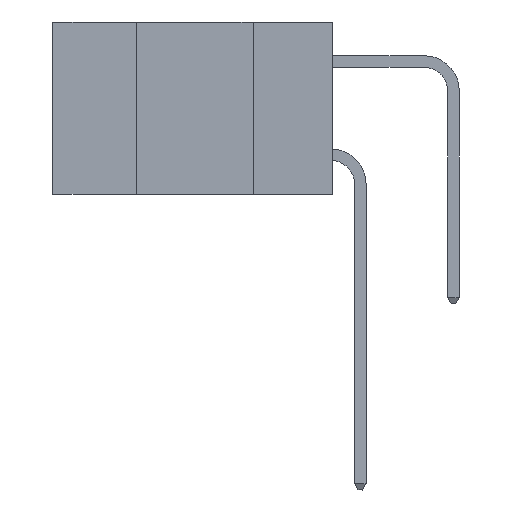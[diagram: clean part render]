
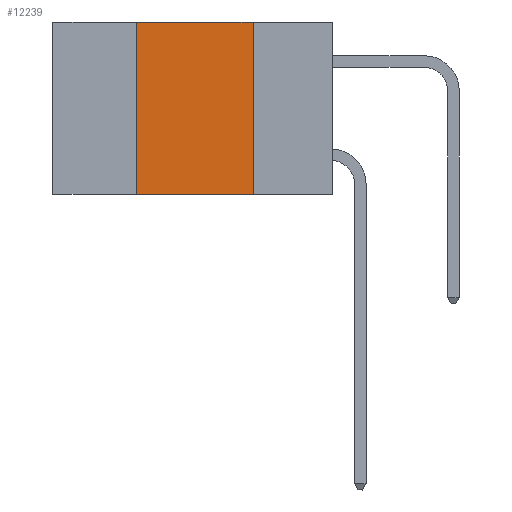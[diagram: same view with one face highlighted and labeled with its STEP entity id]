
A CAD part, left-side view. The second image highlights one B-rep face of the part: STEP entity #12239.
In plain terms, the highlighted planar face has unit normal (-1, 0, 0).
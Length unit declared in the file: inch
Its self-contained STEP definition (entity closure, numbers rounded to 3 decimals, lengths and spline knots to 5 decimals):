
#1234 = LINE ( 'NONE', #1240, #11062 ) ;
#1240 = CARTESIAN_POINT ( 'NONE',  ( 0., 0.6, 0. ) ) ;
#1468 = PLANE ( 'NONE',  #9001 ) ;
#1554 = DIRECTION ( 'NONE',  ( 1., 0., 0. ) ) ;
#2199 = CARTESIAN_POINT ( 'NONE',  ( 0., 0.17, 0. ) ) ;
#2870 = LINE ( 'NONE', #2199, #9507 ) ;
#2906 = CARTESIAN_POINT ( 'NONE',  ( 0., 0.17, 0. ) ) ;
#3190 = DIRECTION ( 'NONE',  ( 0., -1., 0. ) ) ;
#3213 = FACE_OUTER_BOUND ( 'NONE', #6669, .T. ) ;
#3235 = VERTEX_POINT ( 'NONE', #6755 ) ;
#3280 = EDGE_CURVE ( 'NONE', #3368, #3235, #6231, .T. ) ;
#3368 = VERTEX_POINT ( 'NONE', #7272 ) ;
#3686 = VECTOR ( 'NONE', #4241, 39.37008 ) ;
#4083 = LINE ( 'NONE', #10897, #7244 ) ;
#4128 = DIRECTION ( 'NONE',  ( 0., -1., 0. ) ) ;
#4241 = DIRECTION ( 'NONE',  ( 0., 0., 1. ) ) ;
#4661 = CARTESIAN_POINT ( 'NONE',  ( 0., 0.17, -0.37 ) ) ;
#4807 = ORIENTED_EDGE ( 'NONE', *, *, #7144, .F. ) ;
#6231 = LINE ( 'NONE', #9944, #3686 ) ;
#6379 = ORIENTED_EDGE ( 'NONE', *, *, #8574, .F. ) ;
#6669 = EDGE_LOOP ( 'NONE', ( #6379, #4807, #9149, #8578 ) ) ;
#6755 = CARTESIAN_POINT ( 'NONE',  ( 0., 0.42, 0. ) ) ;
#7144 = EDGE_CURVE ( 'NONE', #3235, #11983, #1234, .T. ) ;
#7244 = VECTOR ( 'NONE', #4128, 39.37008 ) ;
#7272 = CARTESIAN_POINT ( 'NONE',  ( 0., 0.42, -0.37 ) ) ;
#7399 = CARTESIAN_POINT ( 'NONE',  ( 0., 0.6, 0. ) ) ;
#8333 = EDGE_CURVE ( 'NONE', #3368, #11503, #4083, .T. ) ;
#8574 = EDGE_CURVE ( 'NONE', #11983, #11503, #2870, .T. ) ;
#8578 = ORIENTED_EDGE ( 'NONE', *, *, #8333, .T. ) ;
#8943 = DIRECTION ( 'NONE',  ( 0., 0., -1. ) ) ;
#9001 = AXIS2_PLACEMENT_3D ( 'NONE', #7399, #1554, #11284 ) ;
#9149 = ORIENTED_EDGE ( 'NONE', *, *, #3280, .F. ) ;
#9507 = VECTOR ( 'NONE', #8943, 39.37008 ) ;
#9944 = CARTESIAN_POINT ( 'NONE',  ( 0., 0.42, 0. ) ) ;
#10897 = CARTESIAN_POINT ( 'NONE',  ( 0., 0.6, -0.37 ) ) ;
#11062 = VECTOR ( 'NONE', #3190, 39.37008 ) ;
#11284 = DIRECTION ( 'NONE',  ( 0., 0., -1. ) ) ;
#11503 = VERTEX_POINT ( 'NONE', #4661 ) ;
#11983 = VERTEX_POINT ( 'NONE', #2906 ) ;
#12239 = ADVANCED_FACE ( 'NONE', ( #3213 ), #1468, .F. ) ;
